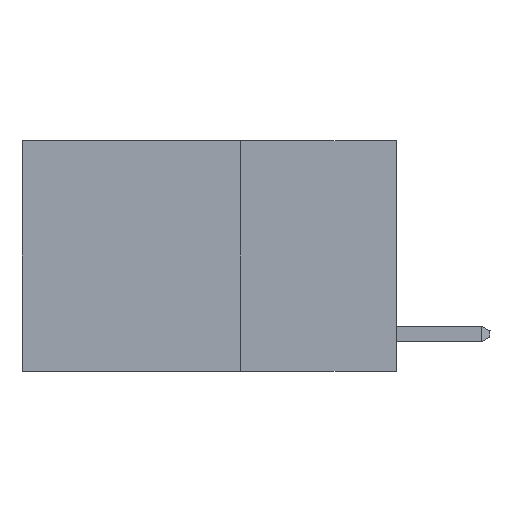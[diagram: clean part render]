
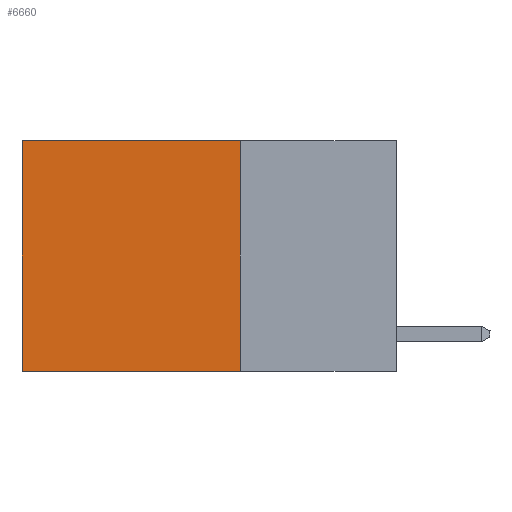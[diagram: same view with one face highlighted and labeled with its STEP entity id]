
A CAD part, left-side view. The second image highlights one B-rep face of the part: STEP entity #6660.
In plain terms, the highlighted planar face has unit normal (-1, 0, 0).
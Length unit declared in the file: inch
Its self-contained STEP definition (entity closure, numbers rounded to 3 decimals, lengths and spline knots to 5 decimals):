
#37 = LINE ( 'NONE', #27576, #23763 ) ;
#2584 = DIRECTION ( 'NONE',  ( 0., 0., -1. ) ) ;
#5070 = VERTEX_POINT ( 'NONE', #24283 ) ;
#5155 = EDGE_CURVE ( 'NONE', #18128, #29738, #27642, .T. ) ;
#5659 = CARTESIAN_POINT ( 'NONE',  ( 0.2625, 0.25, 0. ) ) ;
#5960 = VECTOR ( 'NONE', #21932, 39.37008 ) ;
#6254 = DIRECTION ( 'NONE',  ( 0., 1., 0. ) ) ;
#6315 = ORIENTED_EDGE ( 'NONE', *, *, #29866, .F. ) ;
#6660 = ADVANCED_FACE ( 'NONE', ( #16049 ), #17817, .F. ) ;
#7151 = VECTOR ( 'NONE', #6254, 39.37008 ) ;
#8042 = AXIS2_PLACEMENT_3D ( 'NONE', #5659, #19950, #26593 ) ;
#9333 = LINE ( 'NONE', #27375, #7151 ) ;
#9429 = CARTESIAN_POINT ( 'NONE',  ( 0.2625, 0.6, 0. ) ) ;
#10564 = CARTESIAN_POINT ( 'NONE',  ( 0.2625, 0.25, 0. ) ) ;
#11191 = CARTESIAN_POINT ( 'NONE',  ( 0.2625, 0.6, 0. ) ) ;
#11373 = ORIENTED_EDGE ( 'NONE', *, *, #22632, .F. ) ;
#13319 = EDGE_CURVE ( 'NONE', #15998, #18128, #9333, .T. ) ;
#15796 = DIRECTION ( 'NONE',  ( 0., 1., 0. ) ) ;
#15998 = VERTEX_POINT ( 'NONE', #10564 ) ;
#16049 = FACE_OUTER_BOUND ( 'NONE', #17776, .T. ) ;
#17776 = EDGE_LOOP ( 'NONE', ( #22633, #6315, #11373, #20425 ) ) ;
#17817 = PLANE ( 'NONE',  #8042 ) ;
#18128 = VERTEX_POINT ( 'NONE', #11191 ) ;
#19627 = CARTESIAN_POINT ( 'NONE',  ( 0.2625, 0.6, -0.37 ) ) ;
#19950 = DIRECTION ( 'NONE',  ( 1., 0., 0. ) ) ;
#20425 = ORIENTED_EDGE ( 'NONE', *, *, #13319, .T. ) ;
#21932 = DIRECTION ( 'NONE',  ( 0., 0., -1. ) ) ;
#22632 = EDGE_CURVE ( 'NONE', #15998, #5070, #27776, .T. ) ;
#22633 = ORIENTED_EDGE ( 'NONE', *, *, #5155, .T. ) ;
#23763 = VECTOR ( 'NONE', #15796, 39.37008 ) ;
#24283 = CARTESIAN_POINT ( 'NONE',  ( 0.2625, 0.25, -0.37 ) ) ;
#26593 = DIRECTION ( 'NONE',  ( 0., 0., -1. ) ) ;
#26912 = VECTOR ( 'NONE', #2584, 39.37008 ) ;
#27375 = CARTESIAN_POINT ( 'NONE',  ( 0.2625, 0.25, 0. ) ) ;
#27576 = CARTESIAN_POINT ( 'NONE',  ( 0.2625, 0.25, -0.37 ) ) ;
#27642 = LINE ( 'NONE', #9429, #26912 ) ;
#27776 = LINE ( 'NONE', #29133, #5960 ) ;
#29133 = CARTESIAN_POINT ( 'NONE',  ( 0.2625, 0.25, 0. ) ) ;
#29738 = VERTEX_POINT ( 'NONE', #19627 ) ;
#29866 = EDGE_CURVE ( 'NONE', #5070, #29738, #37, .T. ) ;
